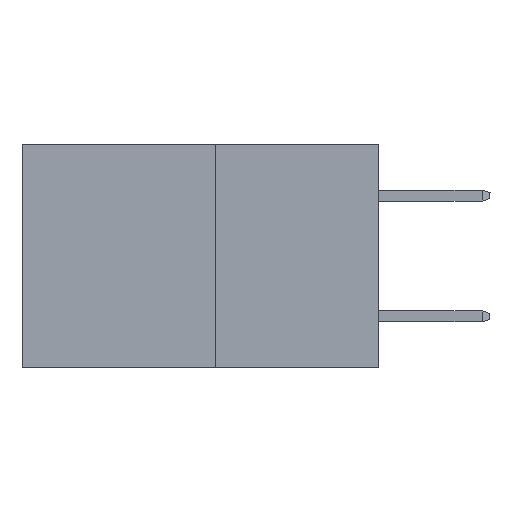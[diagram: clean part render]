
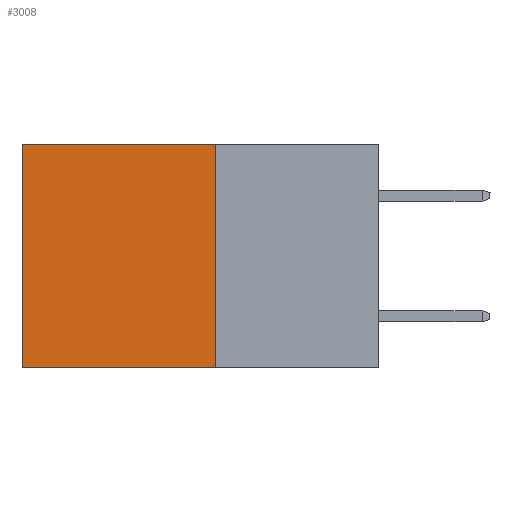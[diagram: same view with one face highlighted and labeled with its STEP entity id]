
A CAD part, left-side view. The second image highlights one B-rep face of the part: STEP entity #3008.
In plain terms, the highlighted planar face has unit normal (-1, 0, 0).
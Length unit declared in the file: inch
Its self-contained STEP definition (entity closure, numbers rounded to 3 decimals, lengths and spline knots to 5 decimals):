
#159 = DIRECTION ( 'NONE',  ( 1., 0., 0. ) ) ;
#845 = FACE_OUTER_BOUND ( 'NONE', #1884, .T. ) ;
#1505 = EDGE_CURVE ( 'NONE', #5684, #10529, #2558, .T. ) ;
#1650 = CARTESIAN_POINT ( 'NONE',  ( 0.277, 0.27, -0.37 ) ) ;
#1884 = EDGE_LOOP ( 'NONE', ( #4042, #4380, #4737, #10030 ) ) ;
#1964 = AXIS2_PLACEMENT_3D ( 'NONE', #1650, #159, #4374 ) ;
#1978 = EDGE_CURVE ( 'NONE', #8957, #10529, #10137, .T. ) ;
#1996 = LINE ( 'NONE', #7393, #6998 ) ;
#2289 = CARTESIAN_POINT ( 'NONE',  ( 0.277, 0.59, -0.37 ) ) ;
#2558 = LINE ( 'NONE', #7479, #7521 ) ;
#3008 = ADVANCED_FACE ( 'NONE', ( #845 ), #5575, .F. ) ;
#4042 = ORIENTED_EDGE ( 'NONE', *, *, #1978, .T. ) ;
#4374 = DIRECTION ( 'NONE',  ( 0., 0., -1. ) ) ;
#4380 = ORIENTED_EDGE ( 'NONE', *, *, #1505, .F. ) ;
#4556 = VERTEX_POINT ( 'NONE', #4825 ) ;
#4737 = ORIENTED_EDGE ( 'NONE', *, *, #8321, .F. ) ;
#4825 = CARTESIAN_POINT ( 'NONE',  ( 0.277, 0.27, 0. ) ) ;
#5575 = PLANE ( 'NONE',  #1964 ) ;
#5684 = VERTEX_POINT ( 'NONE', #10177 ) ;
#6582 = EDGE_CURVE ( 'NONE', #4556, #8957, #1996, .T. ) ;
#6998 = VECTOR ( 'NONE', #7076, 39.37008 ) ;
#7076 = DIRECTION ( 'NONE',  ( 0., 1., 0. ) ) ;
#7393 = CARTESIAN_POINT ( 'NONE',  ( 0.277, 0.27, 0. ) ) ;
#7479 = CARTESIAN_POINT ( 'NONE',  ( 0.277, 0.27, -0.37 ) ) ;
#7521 = VECTOR ( 'NONE', #7759, 39.37008 ) ;
#7568 = LINE ( 'NONE', #10164, #9891 ) ;
#7759 = DIRECTION ( 'NONE',  ( 0., 1., 0. ) ) ;
#7885 = CARTESIAN_POINT ( 'NONE',  ( 0.277, 0.59, -0.37 ) ) ;
#8321 = EDGE_CURVE ( 'NONE', #4556, #5684, #7568, .T. ) ;
#8736 = VECTOR ( 'NONE', #12159, 39.37008 ) ;
#8957 = VERTEX_POINT ( 'NONE', #11994 ) ;
#9891 = VECTOR ( 'NONE', #10136, 39.37008 ) ;
#10030 = ORIENTED_EDGE ( 'NONE', *, *, #6582, .T. ) ;
#10136 = DIRECTION ( 'NONE',  ( 0., 0., -1. ) ) ;
#10137 = LINE ( 'NONE', #7885, #8736 ) ;
#10164 = CARTESIAN_POINT ( 'NONE',  ( 0.277, 0.27, -0.37 ) ) ;
#10177 = CARTESIAN_POINT ( 'NONE',  ( 0.277, 0.27, -0.37 ) ) ;
#10529 = VERTEX_POINT ( 'NONE', #2289 ) ;
#11994 = CARTESIAN_POINT ( 'NONE',  ( 0.277, 0.59, 0. ) ) ;
#12159 = DIRECTION ( 'NONE',  ( 0., 0., -1. ) ) ;
